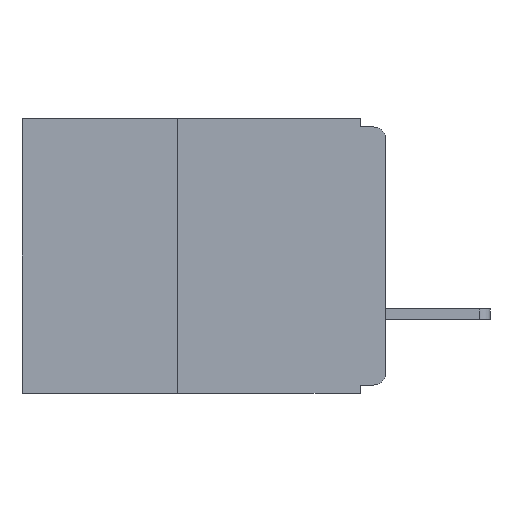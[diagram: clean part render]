
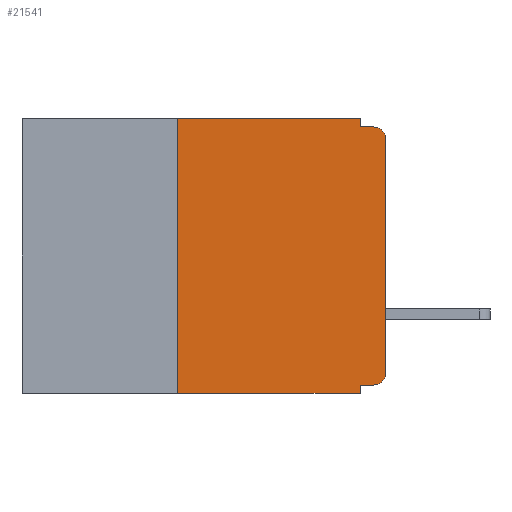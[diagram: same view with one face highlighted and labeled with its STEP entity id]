
A CAD part, left-side view. The second image highlights one B-rep face of the part: STEP entity #21541.
In plain terms, the highlighted planar face has unit normal (-1, 0, 0).
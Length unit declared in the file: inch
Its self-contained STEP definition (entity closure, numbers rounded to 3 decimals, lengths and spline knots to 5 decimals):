
#191 = VERTEX_POINT ( 'NONE', #19989 ) ;
#829 = FACE_OUTER_BOUND ( 'NONE', #10189, .T. ) ;
#1065 = CARTESIAN_POINT ( 'NONE',  ( 0., 0.031, -0.32 ) ) ;
#1072 = EDGE_CURVE ( 'NONE', #19059, #21688, #14944, .T. ) ;
#1422 = VECTOR ( 'NONE', #13586, 39.37008 ) ;
#1773 = VERTEX_POINT ( 'NONE', #24334 ) ;
#1822 = CARTESIAN_POINT ( 'NONE',  ( 0., 0.437, 0. ) ) ;
#1935 = EDGE_CURVE ( 'NONE', #10027, #1773, #15811, .T. ) ;
#2107 = CARTESIAN_POINT ( 'NONE',  ( 0., 0.25, -0.33 ) ) ;
#2674 = ORIENTED_EDGE ( 'NONE', *, *, #13602, .F. ) ;
#3684 = DIRECTION ( 'NONE',  ( 0., 0., -1. ) ) ;
#3881 = ORIENTED_EDGE ( 'NONE', *, *, #1072, .F. ) ;
#3930 = VECTOR ( 'NONE', #16836, 39.37008 ) ;
#4461 = DIRECTION ( 'NONE',  ( 0., -1., 0. ) ) ;
#4908 = CARTESIAN_POINT ( 'NONE',  ( 0., 0., -0.305 ) ) ;
#5210 = DIRECTION ( 'NONE',  ( 0., -1., 0. ) ) ;
#6579 = ORIENTED_EDGE ( 'NONE', *, *, #17885, .F. ) ;
#6670 = EDGE_CURVE ( 'NONE', #17441, #13056, #21258, .T. ) ;
#7218 = ORIENTED_EDGE ( 'NONE', *, *, #7875, .T. ) ;
#7589 = DIRECTION ( 'NONE',  ( 0., 0., -1. ) ) ;
#7628 = AXIS2_PLACEMENT_3D ( 'NONE', #24487, #24481, #24454 ) ;
#7875 = EDGE_CURVE ( 'NONE', #17601, #24675, #13701, .T. ) ;
#7980 = CARTESIAN_POINT ( 'NONE',  ( 0., 0.031, 0. ) ) ;
#8084 = ORIENTED_EDGE ( 'NONE', *, *, #6670, .T. ) ;
#8368 = EDGE_CURVE ( 'NONE', #24675, #17441, #20250, .T. ) ;
#8607 = CARTESIAN_POINT ( 'NONE',  ( 0., 0., -0.025 ) ) ;
#8624 = CARTESIAN_POINT ( 'NONE',  ( 0., 0.25, -0.33 ) ) ;
#9269 = VECTOR ( 'NONE', #5210, 39.37008 ) ;
#10027 = VERTEX_POINT ( 'NONE', #8624 ) ;
#10189 = EDGE_LOOP ( 'NONE', ( #21540, #8084, #6579, #2674, #3881, #16465, #17662, #24566, #11114, #7218 ) ) ;
#10575 = VECTOR ( 'NONE', #4461, 39.37008 ) ;
#10736 = DIRECTION ( 'NONE',  ( 0., 0., -1. ) ) ;
#10797 = AXIS2_PLACEMENT_3D ( 'NONE', #13240, #15162, #3684 ) ;
#10814 = VECTOR ( 'NONE', #10736, 39.37008 ) ;
#11114 = ORIENTED_EDGE ( 'NONE', *, *, #19303, .F. ) ;
#11401 = LINE ( 'NONE', #18437, #10814 ) ;
#13056 = VERTEX_POINT ( 'NONE', #20547 ) ;
#13240 = CARTESIAN_POINT ( 'NONE',  ( 0., 0.437, 0. ) ) ;
#13586 = DIRECTION ( 'NONE',  ( 0., 0., 1. ) ) ;
#13602 = EDGE_CURVE ( 'NONE', #21688, #191, #11401, .T. ) ;
#13701 = CIRCLE ( 'NONE', #7628, 0.015 ) ;
#14108 = LINE ( 'NONE', #15000, #3930 ) ;
#14942 = EDGE_CURVE ( 'NONE', #23766, #1773, #19148, .T. ) ;
#14944 = LINE ( 'NONE', #1822, #9269 ) ;
#15000 = CARTESIAN_POINT ( 'NONE',  ( 0., 0., -0.32 ) ) ;
#15060 = EDGE_CURVE ( 'NONE', #10027, #19059, #22397, .T. ) ;
#15162 = DIRECTION ( 'NONE',  ( 1., 0., 0. ) ) ;
#15723 = DIRECTION ( 'NONE',  ( 0., 0., -1. ) ) ;
#15783 = DIRECTION ( 'NONE',  ( -1., 0., 0. ) ) ;
#15811 = LINE ( 'NONE', #22513, #20917 ) ;
#15839 = CARTESIAN_POINT ( 'NONE',  ( 0., 0.015, -0.025 ) ) ;
#16465 = ORIENTED_EDGE ( 'NONE', *, *, #15060, .F. ) ;
#16836 = DIRECTION ( 'NONE',  ( 0., 1., 0. ) ) ;
#17092 = CARTESIAN_POINT ( 'NONE',  ( 0., 0.031, -0.33 ) ) ;
#17441 = VERTEX_POINT ( 'NONE', #8607 ) ;
#17601 = VERTEX_POINT ( 'NONE', #20811 ) ;
#17662 = ORIENTED_EDGE ( 'NONE', *, *, #1935, .T. ) ;
#17867 = CARTESIAN_POINT ( 'NONE',  ( 0., 0., -0.01 ) ) ;
#17885 = EDGE_CURVE ( 'NONE', #191, #13056, #21351, .T. ) ;
#18124 = DIRECTION ( 'NONE',  ( 0., 0., 1. ) ) ;
#18272 = CARTESIAN_POINT ( 'NONE',  ( 0., 0., 0. ) ) ;
#18437 = CARTESIAN_POINT ( 'NONE',  ( 0., 0.031, 0. ) ) ;
#19059 = VERTEX_POINT ( 'NONE', #20045 ) ;
#19148 = LINE ( 'NONE', #17092, #23595 ) ;
#19303 = EDGE_CURVE ( 'NONE', #17601, #23766, #14108, .T. ) ;
#19989 = CARTESIAN_POINT ( 'NONE',  ( 0., 0.031, -0.01 ) ) ;
#20045 = CARTESIAN_POINT ( 'NONE',  ( 0., 0.25, 0. ) ) ;
#20250 = LINE ( 'NONE', #18272, #24738 ) ;
#20258 = AXIS2_PLACEMENT_3D ( 'NONE', #15839, #15783, #15723 ) ;
#20547 = CARTESIAN_POINT ( 'NONE',  ( 0., 0.015, -0.01 ) ) ;
#20811 = CARTESIAN_POINT ( 'NONE',  ( 0., 0.015, -0.32 ) ) ;
#20917 = VECTOR ( 'NONE', #22568, 39.37008 ) ;
#21258 = CIRCLE ( 'NONE', #20258, 0.015 ) ;
#21351 = LINE ( 'NONE', #17867, #10575 ) ;
#21540 = ORIENTED_EDGE ( 'NONE', *, *, #8368, .T. ) ;
#21541 = ADVANCED_FACE ( 'NONE', ( #829 ), #24704, .F. ) ;
#21688 = VERTEX_POINT ( 'NONE', #7980 ) ;
#22397 = LINE ( 'NONE', #2107, #1422 ) ;
#22513 = CARTESIAN_POINT ( 'NONE',  ( 0., 0.437, -0.33 ) ) ;
#22568 = DIRECTION ( 'NONE',  ( 0., -1., 0. ) ) ;
#23595 = VECTOR ( 'NONE', #7589, 39.37008 ) ;
#23766 = VERTEX_POINT ( 'NONE', #1065 ) ;
#24334 = CARTESIAN_POINT ( 'NONE',  ( 0., 0.031, -0.33 ) ) ;
#24454 = DIRECTION ( 'NONE',  ( 0., 0., -1. ) ) ;
#24481 = DIRECTION ( 'NONE',  ( -1., 0., 0. ) ) ;
#24487 = CARTESIAN_POINT ( 'NONE',  ( 0., 0.015, -0.305 ) ) ;
#24566 = ORIENTED_EDGE ( 'NONE', *, *, #14942, .F. ) ;
#24675 = VERTEX_POINT ( 'NONE', #4908 ) ;
#24704 = PLANE ( 'NONE',  #10797 ) ;
#24738 = VECTOR ( 'NONE', #18124, 39.37008 ) ;
